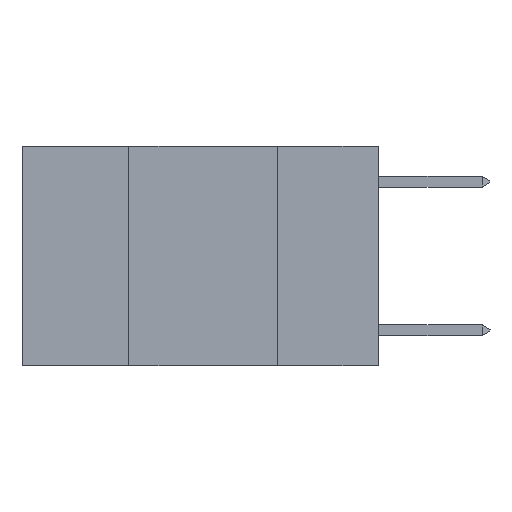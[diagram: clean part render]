
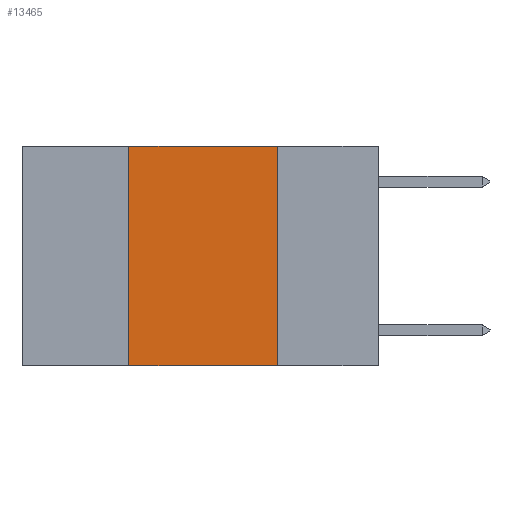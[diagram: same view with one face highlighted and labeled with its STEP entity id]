
A CAD part, left-side view. The second image highlights one B-rep face of the part: STEP entity #13465.
In plain terms, the highlighted planar face has unit normal (-1, 0, 0).
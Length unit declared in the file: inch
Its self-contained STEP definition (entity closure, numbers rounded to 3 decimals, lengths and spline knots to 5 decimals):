
#76 = CARTESIAN_POINT ( 'NONE',  ( 0., 0.6, 0. ) ) ;
#724 = DIRECTION ( 'NONE',  ( 0., 0., -1. ) ) ;
#1749 = DIRECTION ( 'NONE',  ( 0., 0., -1. ) ) ;
#2642 = FACE_OUTER_BOUND ( 'NONE', #19491, .T. ) ;
#2714 = EDGE_CURVE ( 'NONE', #15070, #13042, #5645, .T. ) ;
#3182 = VERTEX_POINT ( 'NONE', #5294 ) ;
#3936 = EDGE_CURVE ( 'NONE', #14124, #15070, #8483, .T. ) ;
#4049 = ORIENTED_EDGE ( 'NONE', *, *, #19709, .T. ) ;
#4439 = DIRECTION ( 'NONE',  ( 0., -1., 0. ) ) ;
#5016 = EDGE_CURVE ( 'NONE', #13042, #3182, #9677, .T. ) ;
#5109 = LINE ( 'NONE', #12129, #12825 ) ;
#5294 = CARTESIAN_POINT ( 'NONE',  ( 0., 0.17, -0.37 ) ) ;
#5326 = CARTESIAN_POINT ( 'NONE',  ( 0., 0.42, -0.37 ) ) ;
#5645 = LINE ( 'NONE', #12065, #17377 ) ;
#6036 = VECTOR ( 'NONE', #724, 39.37008 ) ;
#6929 = CARTESIAN_POINT ( 'NONE',  ( 0., 0.17, 0. ) ) ;
#7751 = CARTESIAN_POINT ( 'NONE',  ( 0., 0.42, 0. ) ) ;
#8483 = LINE ( 'NONE', #14687, #8973 ) ;
#8973 = VECTOR ( 'NONE', #17689, 39.37008 ) ;
#9677 = LINE ( 'NONE', #16311, #6036 ) ;
#11126 = DIRECTION ( 'NONE',  ( 1., 0., 0. ) ) ;
#12065 = CARTESIAN_POINT ( 'NONE',  ( 0., 0.6, 0. ) ) ;
#12129 = CARTESIAN_POINT ( 'NONE',  ( 0., 0.6, -0.37 ) ) ;
#12825 = VECTOR ( 'NONE', #15114, 39.37008 ) ;
#13042 = VERTEX_POINT ( 'NONE', #6929 ) ;
#13465 = ADVANCED_FACE ( 'NONE', ( #2642 ), #14159, .F. ) ;
#13587 = ORIENTED_EDGE ( 'NONE', *, *, #3936, .F. ) ;
#14124 = VERTEX_POINT ( 'NONE', #5326 ) ;
#14159 = PLANE ( 'NONE',  #14464 ) ;
#14464 = AXIS2_PLACEMENT_3D ( 'NONE', #76, #11126, #1749 ) ;
#14687 = CARTESIAN_POINT ( 'NONE',  ( 0., 0.42, 0. ) ) ;
#15070 = VERTEX_POINT ( 'NONE', #7751 ) ;
#15114 = DIRECTION ( 'NONE',  ( 0., -1., 0. ) ) ;
#16311 = CARTESIAN_POINT ( 'NONE',  ( 0., 0.17, 0. ) ) ;
#17303 = ORIENTED_EDGE ( 'NONE', *, *, #2714, .F. ) ;
#17377 = VECTOR ( 'NONE', #4439, 39.37008 ) ;
#17689 = DIRECTION ( 'NONE',  ( 0., 0., 1. ) ) ;
#18925 = ORIENTED_EDGE ( 'NONE', *, *, #5016, .F. ) ;
#19491 = EDGE_LOOP ( 'NONE', ( #18925, #17303, #13587, #4049 ) ) ;
#19709 = EDGE_CURVE ( 'NONE', #14124, #3182, #5109, .T. ) ;
